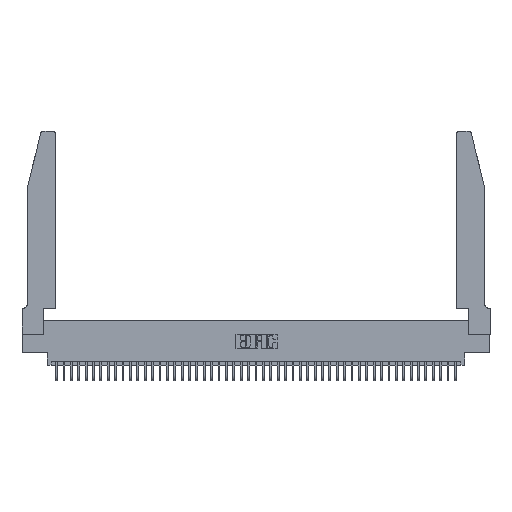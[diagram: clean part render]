
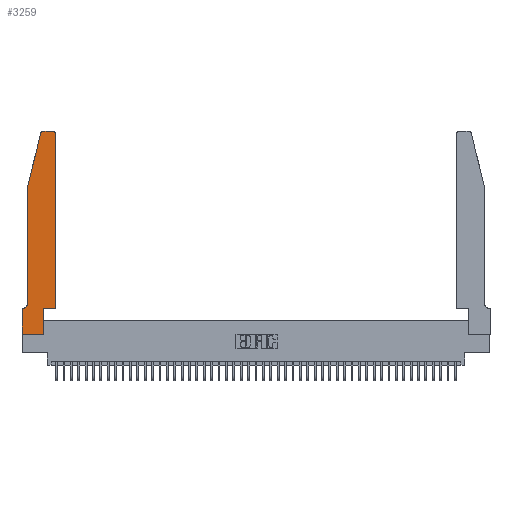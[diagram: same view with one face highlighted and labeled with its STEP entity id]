
A CAD part, top view. The second image highlights one B-rep face of the part: STEP entity #3259.
In plain terms, the highlighted planar face has unit normal (0, 0, 1).
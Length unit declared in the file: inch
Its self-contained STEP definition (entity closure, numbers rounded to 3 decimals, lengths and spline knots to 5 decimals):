
#135 = EDGE_CURVE ( 'NONE', #24716, #11457, #3190, .T. ) ;
#910 = DIRECTION ( 'NONE',  ( 0., -1., 0. ) ) ;
#1122 = VERTEX_POINT ( 'NONE', #8742 ) ;
#1516 = CARTESIAN_POINT ( 'NONE',  ( 0.0755, 2., 0.37 ) ) ;
#1718 = VECTOR ( 'NONE', #27482, 39.37008 ) ;
#1932 = CARTESIAN_POINT ( 'NONE',  ( 0.2865, 0.35, 0.37 ) ) ;
#2272 = DIRECTION ( 'NONE',  ( 1., 0., 0. ) ) ;
#2681 = CARTESIAN_POINT ( 'NONE',  ( 0.284, 2.75, 0.37 ) ) ;
#2789 = ORIENTED_EDGE ( 'NONE', *, *, #36252, .T. ) ;
#3190 = LINE ( 'NONE', #19674, #33901 ) ;
#3259 = ADVANCED_FACE ( 'NONE', ( #12944 ), #46685, .T. ) ;
#3326 = VECTOR ( 'NONE', #26285, 39.37008 ) ;
#3861 = LINE ( 'NONE', #44764, #3326 ) ;
#4023 = EDGE_LOOP ( 'NONE', ( #14736, #35608, #26660, #33191, #46276, #2789, #24363, #31451, #14418, #19254, #21081, #41901 ) ) ;
#4142 = LINE ( 'NONE', #5237, #15180 ) ;
#5193 = LINE ( 'NONE', #24077, #1718 ) ;
#5237 = CARTESIAN_POINT ( 'NONE',  ( 0.4505, 0.35, 0.37 ) ) ;
#5517 = AXIS2_PLACEMENT_3D ( 'NONE', #17331, #46524, #2272 ) ;
#5597 = VERTEX_POINT ( 'NONE', #18712 ) ;
#6832 = CARTESIAN_POINT ( 'NONE',  ( 0.4205, 2.75, 0.37 ) ) ;
#8091 = VECTOR ( 'NONE', #8498, 39.37008 ) ;
#8370 = CIRCLE ( 'NONE', #23627, 0.03 ) ;
#8498 = DIRECTION ( 'NONE',  ( -1., 0., 0. ) ) ;
#8547 = VERTEX_POINT ( 'NONE', #2681 ) ;
#8728 = EDGE_CURVE ( 'NONE', #5597, #24716, #5193, .T. ) ;
#8742 = CARTESIAN_POINT ( 'NONE',  ( 0.0755, 0.42, 0.37 ) ) ;
#8805 = CARTESIAN_POINT ( 'NONE',  ( 0.2605, 2.75, 0.37 ) ) ;
#8832 = LINE ( 'NONE', #1932, #27960 ) ;
#9894 = EDGE_CURVE ( 'NONE', #20188, #20814, #29988, .T. ) ;
#11457 = VERTEX_POINT ( 'NONE', #35006 ) ;
#12293 = EDGE_CURVE ( 'NONE', #20814, #1122, #41884, .T. ) ;
#12944 = FACE_OUTER_BOUND ( 'NONE', #4023, .T. ) ;
#14322 = CARTESIAN_POINT ( 'NONE',  ( 0.2865, 0.35, 0.37 ) ) ;
#14418 = ORIENTED_EDGE ( 'NONE', *, *, #44852, .T. ) ;
#14736 = ORIENTED_EDGE ( 'NONE', *, *, #32825, .T. ) ;
#15180 = VECTOR ( 'NONE', #35226, 39.37008 ) ;
#16263 = DIRECTION ( 'NONE',  ( -1., 0., 0. ) ) ;
#16337 = EDGE_CURVE ( 'NONE', #1122, #21755, #40625, .T. ) ;
#17331 = CARTESIAN_POINT ( 'NONE',  ( 0., 0.35, 0.37 ) ) ;
#17363 = LINE ( 'NONE', #38283, #8091 ) ;
#18513 = DIRECTION ( 'NONE',  ( 1., 0., 0. ) ) ;
#18712 = CARTESIAN_POINT ( 'NONE',  ( 0., 0.35, 0.37 ) ) ;
#19254 = ORIENTED_EDGE ( 'NONE', *, *, #41267, .T. ) ;
#19674 = CARTESIAN_POINT ( 'NONE',  ( 0., 0., 0.37 ) ) ;
#20188 = VERTEX_POINT ( 'NONE', #23700 ) ;
#20814 = VERTEX_POINT ( 'NONE', #1516 ) ;
#21081 = ORIENTED_EDGE ( 'NONE', *, *, #35297, .T. ) ;
#21499 = CARTESIAN_POINT ( 'NONE',  ( 0.4205, 2.72, 0.37 ) ) ;
#21755 = VERTEX_POINT ( 'NONE', #31465 ) ;
#21774 = LINE ( 'NONE', #8805, #22371 ) ;
#21944 = DIRECTION ( 'NONE',  ( -0.239, -0.971, 0. ) ) ;
#22371 = VECTOR ( 'NONE', #16263, 39.37008 ) ;
#22784 = CARTESIAN_POINT ( 'NONE',  ( 0., 0., 0.37 ) ) ;
#23627 = AXIS2_PLACEMENT_3D ( 'NONE', #37299, #33736, #18513 ) ;
#23700 = CARTESIAN_POINT ( 'NONE',  ( 0.25487, 2.72718, 0.37 ) ) ;
#24077 = CARTESIAN_POINT ( 'NONE',  ( 0., 0., 0.37 ) ) ;
#24363 = ORIENTED_EDGE ( 'NONE', *, *, #8728, .T. ) ;
#24716 = VERTEX_POINT ( 'NONE', #22784 ) ;
#25530 = CARTESIAN_POINT ( 'NONE',  ( 0.0755, 2., 0.37 ) ) ;
#26242 = EDGE_CURVE ( 'NONE', #30450, #40455, #36505, .T. ) ;
#26285 = DIRECTION ( 'NONE',  ( 1., 0., 0. ) ) ;
#26660 = ORIENTED_EDGE ( 'NONE', *, *, #9894, .T. ) ;
#27000 = DIRECTION ( 'NONE',  ( 1., 0., 0. ) ) ;
#27461 = EDGE_CURVE ( 'NONE', #8547, #20188, #8370, .T. ) ;
#27482 = DIRECTION ( 'NONE',  ( 0., -1., 0. ) ) ;
#27960 = VECTOR ( 'NONE', #35610, 39.37008 ) ;
#29140 = DIRECTION ( 'NONE',  ( 0., 0., 1. ) ) ;
#29445 = DIRECTION ( 'NONE',  ( 1., 0., 0. ) ) ;
#29988 = LINE ( 'NONE', #25530, #46831 ) ;
#30450 = VERTEX_POINT ( 'NONE', #33836 ) ;
#30907 = CARTESIAN_POINT ( 'NONE',  ( 0.0755, 2., 0.37 ) ) ;
#30987 = AXIS2_PLACEMENT_3D ( 'NONE', #39628, #35800, #36267 ) ;
#31451 = ORIENTED_EDGE ( 'NONE', *, *, #135, .T. ) ;
#31465 = CARTESIAN_POINT ( 'NONE',  ( 0.0055, 0.35, 0.37 ) ) ;
#32087 = VECTOR ( 'NONE', #910, 39.37008 ) ;
#32825 = EDGE_CURVE ( 'NONE', #40455, #8547, #21774, .T. ) ;
#33191 = ORIENTED_EDGE ( 'NONE', *, *, #12293, .T. ) ;
#33669 = VERTEX_POINT ( 'NONE', #14322 ) ;
#33736 = DIRECTION ( 'NONE',  ( 0., 0., 1. ) ) ;
#33836 = CARTESIAN_POINT ( 'NONE',  ( 0.4505, 2.72, 0.37 ) ) ;
#33901 = VECTOR ( 'NONE', #27000, 39.37008 ) ;
#35006 = CARTESIAN_POINT ( 'NONE',  ( 0.2865, 0., 0.37 ) ) ;
#35226 = DIRECTION ( 'NONE',  ( 0., 1., 0. ) ) ;
#35297 = EDGE_CURVE ( 'NONE', #44453, #30450, #4142, .T. ) ;
#35608 = ORIENTED_EDGE ( 'NONE', *, *, #27461, .T. ) ;
#35610 = DIRECTION ( 'NONE',  ( 0., 1., 0. ) ) ;
#35800 = DIRECTION ( 'NONE',  ( 0., 0., -1. ) ) ;
#36252 = EDGE_CURVE ( 'NONE', #21755, #5597, #17363, .T. ) ;
#36267 = DIRECTION ( 'NONE',  ( -1., 0., 0. ) ) ;
#36505 = CIRCLE ( 'NONE', #38193, 0.03 ) ;
#37299 = CARTESIAN_POINT ( 'NONE',  ( 0.284, 2.72, 0.37 ) ) ;
#38193 = AXIS2_PLACEMENT_3D ( 'NONE', #21499, #29140, #29445 ) ;
#38283 = CARTESIAN_POINT ( 'NONE',  ( 0.0755, 0.35, 0.37 ) ) ;
#39628 = CARTESIAN_POINT ( 'NONE',  ( 0.0055, 0.42, 0.37 ) ) ;
#40455 = VERTEX_POINT ( 'NONE', #6832 ) ;
#40495 = CARTESIAN_POINT ( 'NONE',  ( 0.4505, 0.35, 0.37 ) ) ;
#40625 = CIRCLE ( 'NONE', #30987, 0.07 ) ;
#41267 = EDGE_CURVE ( 'NONE', #33669, #44453, #3861, .T. ) ;
#41884 = LINE ( 'NONE', #30907, #32087 ) ;
#41901 = ORIENTED_EDGE ( 'NONE', *, *, #26242, .T. ) ;
#44453 = VERTEX_POINT ( 'NONE', #40495 ) ;
#44764 = CARTESIAN_POINT ( 'NONE',  ( 0.4505, 0.35, 0.37 ) ) ;
#44852 = EDGE_CURVE ( 'NONE', #11457, #33669, #8832, .T. ) ;
#46276 = ORIENTED_EDGE ( 'NONE', *, *, #16337, .T. ) ;
#46524 = DIRECTION ( 'NONE',  ( 0., 0., 1. ) ) ;
#46685 = PLANE ( 'NONE',  #5517 ) ;
#46831 = VECTOR ( 'NONE', #21944, 39.37008 ) ;
